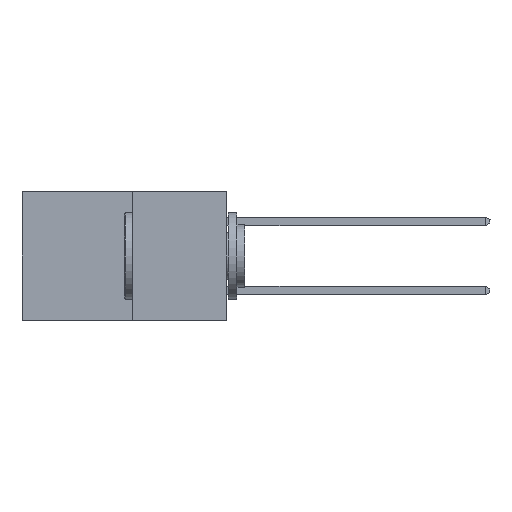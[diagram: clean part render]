
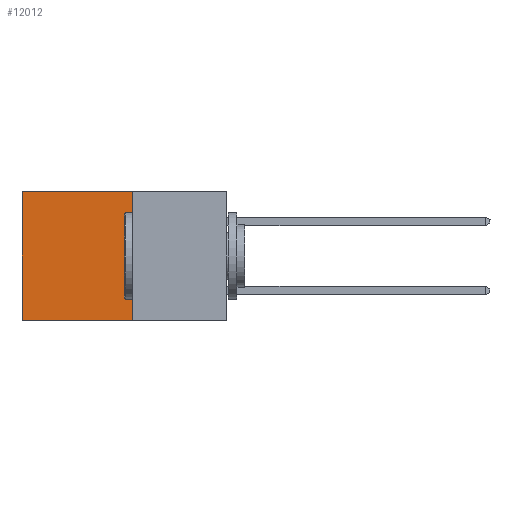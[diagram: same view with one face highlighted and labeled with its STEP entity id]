
A CAD part, left-side view. The second image highlights one B-rep face of the part: STEP entity #12012.
In plain terms, the highlighted planar face has unit normal (-1, 0, 0).
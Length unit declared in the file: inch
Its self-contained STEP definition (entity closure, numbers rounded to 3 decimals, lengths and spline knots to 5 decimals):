
#136 = ORIENTED_EDGE ( 'NONE', *, *, #3546, .F. ) ;
#371 = CARTESIAN_POINT ( 'NONE',  ( 0.277, 0.27, 0. ) ) ;
#885 = LINE ( 'NONE', #15788, #4669 ) ;
#1644 = LINE ( 'NONE', #13708, #8031 ) ;
#2109 = VERTEX_POINT ( 'NONE', #9524 ) ;
#2501 = EDGE_CURVE ( 'NONE', #9368, #2109, #10514, .T. ) ;
#2697 = VECTOR ( 'NONE', #15350, 39.37008 ) ;
#3546 = EDGE_CURVE ( 'NONE', #3984, #9368, #1644, .T. ) ;
#3904 = ORIENTED_EDGE ( 'NONE', *, *, #10198, .T. ) ;
#3984 = VERTEX_POINT ( 'NONE', #371 ) ;
#4139 = CARTESIAN_POINT ( 'NONE',  ( 0.277, 0.27, -0.37 ) ) ;
#4611 = CARTESIAN_POINT ( 'NONE',  ( 0.277, 0.27, -0.37 ) ) ;
#4669 = VECTOR ( 'NONE', #15841, 39.37008 ) ;
#5407 = DIRECTION ( 'NONE',  ( 1., 0., 0. ) ) ;
#5497 = EDGE_LOOP ( 'NONE', ( #9525, #9940, #136, #3904 ) ) ;
#5700 = CARTESIAN_POINT ( 'NONE',  ( 0.277, 0.59, 0. ) ) ;
#6131 = VERTEX_POINT ( 'NONE', #5700 ) ;
#8031 = VECTOR ( 'NONE', #15382, 39.37008 ) ;
#8871 = EDGE_CURVE ( 'NONE', #6131, #2109, #9932, .T. ) ;
#9232 = FACE_OUTER_BOUND ( 'NONE', #5497, .T. ) ;
#9368 = VERTEX_POINT ( 'NONE', #9848 ) ;
#9524 = CARTESIAN_POINT ( 'NONE',  ( 0.277, 0.59, -0.37 ) ) ;
#9525 = ORIENTED_EDGE ( 'NONE', *, *, #8871, .T. ) ;
#9848 = CARTESIAN_POINT ( 'NONE',  ( 0.277, 0.27, -0.37 ) ) ;
#9932 = LINE ( 'NONE', #12782, #2697 ) ;
#9940 = ORIENTED_EDGE ( 'NONE', *, *, #2501, .F. ) ;
#10198 = EDGE_CURVE ( 'NONE', #3984, #6131, #885, .T. ) ;
#10514 = LINE ( 'NONE', #4611, #16515 ) ;
#10617 = DIRECTION ( 'NONE',  ( 0., 1., 0. ) ) ;
#11895 = PLANE ( 'NONE',  #12856 ) ;
#12012 = ADVANCED_FACE ( 'NONE', ( #9232 ), #11895, .F. ) ;
#12782 = CARTESIAN_POINT ( 'NONE',  ( 0.277, 0.59, -0.37 ) ) ;
#12856 = AXIS2_PLACEMENT_3D ( 'NONE', #4139, #5407, #14432 ) ;
#13708 = CARTESIAN_POINT ( 'NONE',  ( 0.277, 0.27, -0.37 ) ) ;
#14432 = DIRECTION ( 'NONE',  ( 0., 0., -1. ) ) ;
#15350 = DIRECTION ( 'NONE',  ( 0., 0., -1. ) ) ;
#15382 = DIRECTION ( 'NONE',  ( 0., 0., -1. ) ) ;
#15788 = CARTESIAN_POINT ( 'NONE',  ( 0.277, 0.27, 0. ) ) ;
#15841 = DIRECTION ( 'NONE',  ( 0., 1., 0. ) ) ;
#16515 = VECTOR ( 'NONE', #10617, 39.37008 ) ;
